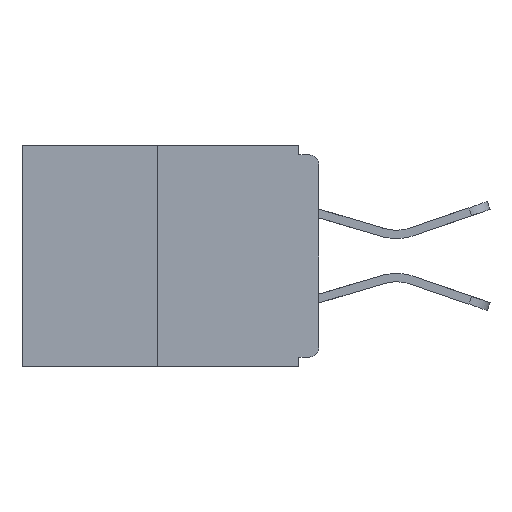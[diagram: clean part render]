
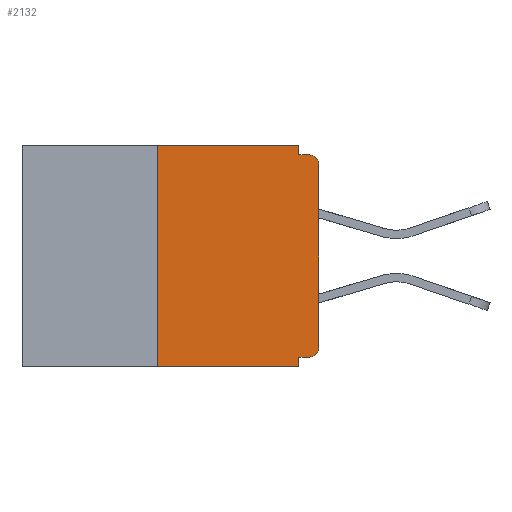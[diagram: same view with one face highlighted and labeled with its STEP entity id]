
A CAD part, left-side view. The second image highlights one B-rep face of the part: STEP entity #2132.
In plain terms, the highlighted planar face has unit normal (-1, 0, 0).
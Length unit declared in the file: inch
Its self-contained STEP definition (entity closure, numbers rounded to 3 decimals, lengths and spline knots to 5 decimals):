
#478 = ORIENTED_EDGE ( 'NONE', *, *, #6027, .F. ) ;
#513 = CARTESIAN_POINT ( 'NONE',  ( 0., 0., 0. ) ) ;
#827 = CARTESIAN_POINT ( 'NONE',  ( 0., 0.031, 0. ) ) ;
#1847 = CARTESIAN_POINT ( 'NONE',  ( 0., 0., -0.328 ) ) ;
#2132 = ADVANCED_FACE ( 'NONE', ( #8155 ), #9119, .F. ) ;
#2472 = ORIENTED_EDGE ( 'NONE', *, *, #11041, .F. ) ;
#3464 = CARTESIAN_POINT ( 'NONE',  ( 0., 0.46, 0. ) ) ;
#3646 = CARTESIAN_POINT ( 'NONE',  ( 0., 0.031, -0.015 ) ) ;
#4308 = VECTOR ( 'NONE', #7801, 39.37008 ) ;
#4330 = LINE ( 'NONE', #12150, #16354 ) ;
#4912 = EDGE_CURVE ( 'NONE', #11261, #14830, #19458, .T. ) ;
#5248 = ORIENTED_EDGE ( 'NONE', *, *, #5717, .F. ) ;
#5266 = LINE ( 'NONE', #8279, #11574 ) ;
#5592 = CARTESIAN_POINT ( 'NONE',  ( 0., 0.46, 0. ) ) ;
#5676 = DIRECTION ( 'NONE',  ( 0., -1., 0. ) ) ;
#5717 = EDGE_CURVE ( 'NONE', #6964, #14830, #18821, .T. ) ;
#6027 = EDGE_CURVE ( 'NONE', #24939, #6964, #5266, .T. ) ;
#6182 = DIRECTION ( 'NONE',  ( 0., 0., -1. ) ) ;
#6317 = DIRECTION ( 'NONE',  ( 0., 0., 1. ) ) ;
#6696 = VERTEX_POINT ( 'NONE', #16101 ) ;
#6715 = LINE ( 'NONE', #23277, #4308 ) ;
#6763 = DIRECTION ( 'NONE',  ( -1., 0., 0. ) ) ;
#6900 = VERTEX_POINT ( 'NONE', #21086 ) ;
#6964 = VERTEX_POINT ( 'NONE', #3646 ) ;
#7274 = DIRECTION ( 'NONE',  ( 0., 0., -1. ) ) ;
#7403 = VECTOR ( 'NONE', #16596, 39.37008 ) ;
#7737 = ORIENTED_EDGE ( 'NONE', *, *, #10737, .T. ) ;
#7801 = DIRECTION ( 'NONE',  ( 0., -1., 0. ) ) ;
#8001 = DIRECTION ( 'NONE',  ( 0., 0., -1. ) ) ;
#8126 = DIRECTION ( 'NONE',  ( 0., 0., -1. ) ) ;
#8155 = FACE_OUTER_BOUND ( 'NONE', #24048, .T. ) ;
#8279 = CARTESIAN_POINT ( 'NONE',  ( 0., 0.031, 0. ) ) ;
#8418 = VERTEX_POINT ( 'NONE', #11723 ) ;
#8738 = ORIENTED_EDGE ( 'NONE', *, *, #9827, .F. ) ;
#8752 = EDGE_CURVE ( 'NONE', #11117, #6696, #12344, .T. ) ;
#8955 = CARTESIAN_POINT ( 'NONE',  ( 0., 0., -0.015 ) ) ;
#9119 = PLANE ( 'NONE',  #12681 ) ;
#9827 = EDGE_CURVE ( 'NONE', #15967, #6900, #18626, .T. ) ;
#10737 = EDGE_CURVE ( 'NONE', #11117, #8418, #11955, .T. ) ;
#10884 = ORIENTED_EDGE ( 'NONE', *, *, #18009, .F. ) ;
#10940 = CARTESIAN_POINT ( 'NONE',  ( 0., 0.25, -0.343 ) ) ;
#11041 = EDGE_CURVE ( 'NONE', #6900, #24939, #11637, .T. ) ;
#11117 = VERTEX_POINT ( 'NONE', #15347 ) ;
#11261 = VERTEX_POINT ( 'NONE', #15743 ) ;
#11399 = VECTOR ( 'NONE', #14723, 39.37008 ) ;
#11574 = VECTOR ( 'NONE', #6182, 39.37008 ) ;
#11637 = LINE ( 'NONE', #5592, #21295 ) ;
#11723 = CARTESIAN_POINT ( 'NONE',  ( 0., 0., -0.313 ) ) ;
#11955 = CIRCLE ( 'NONE', #20068, 0.015 ) ;
#12150 = CARTESIAN_POINT ( 'NONE',  ( 0., 0.031, -0.343 ) ) ;
#12343 = LINE ( 'NONE', #513, #22923 ) ;
#12344 = LINE ( 'NONE', #1847, #23828 ) ;
#12681 = AXIS2_PLACEMENT_3D ( 'NONE', #3464, #12968, #7274 ) ;
#12968 = DIRECTION ( 'NONE',  ( 1., 0., 0. ) ) ;
#14162 = CARTESIAN_POINT ( 'NONE',  ( 0., 0.015, -0.313 ) ) ;
#14723 = DIRECTION ( 'NONE',  ( 0., 0., 1. ) ) ;
#14830 = VERTEX_POINT ( 'NONE', #24070 ) ;
#15347 = CARTESIAN_POINT ( 'NONE',  ( 0., 0.015, -0.328 ) ) ;
#15743 = CARTESIAN_POINT ( 'NONE',  ( 0., 0., -0.03 ) ) ;
#15967 = VERTEX_POINT ( 'NONE', #10940 ) ;
#16101 = CARTESIAN_POINT ( 'NONE',  ( 0., 0.031, -0.328 ) ) ;
#16354 = VECTOR ( 'NONE', #8126, 39.37008 ) ;
#16596 = DIRECTION ( 'NONE',  ( 0., -1., 0. ) ) ;
#17575 = AXIS2_PLACEMENT_3D ( 'NONE', #21307, #19428, #8001 ) ;
#17895 = EDGE_CURVE ( 'NONE', #15967, #18584, #6715, .T. ) ;
#18009 = EDGE_CURVE ( 'NONE', #6696, #18584, #4330, .T. ) ;
#18130 = ORIENTED_EDGE ( 'NONE', *, *, #19625, .T. ) ;
#18584 = VERTEX_POINT ( 'NONE', #20282 ) ;
#18610 = ORIENTED_EDGE ( 'NONE', *, *, #8752, .F. ) ;
#18626 = LINE ( 'NONE', #20621, #11399 ) ;
#18821 = LINE ( 'NONE', #8955, #7403 ) ;
#19428 = DIRECTION ( 'NONE',  ( -1., 0., 0. ) ) ;
#19458 = CIRCLE ( 'NONE', #17575, 0.015 ) ;
#19483 = ORIENTED_EDGE ( 'NONE', *, *, #4912, .T. ) ;
#19625 = EDGE_CURVE ( 'NONE', #8418, #11261, #12343, .T. ) ;
#20068 = AXIS2_PLACEMENT_3D ( 'NONE', #14162, #6763, #20220 ) ;
#20220 = DIRECTION ( 'NONE',  ( 0., 0., -1. ) ) ;
#20282 = CARTESIAN_POINT ( 'NONE',  ( 0., 0.031, -0.343 ) ) ;
#20621 = CARTESIAN_POINT ( 'NONE',  ( 0., 0.25, 0. ) ) ;
#21086 = CARTESIAN_POINT ( 'NONE',  ( 0., 0.25, 0. ) ) ;
#21295 = VECTOR ( 'NONE', #5676, 39.37008 ) ;
#21307 = CARTESIAN_POINT ( 'NONE',  ( 0., 0.015, -0.03 ) ) ;
#21974 = ORIENTED_EDGE ( 'NONE', *, *, #17895, .T. ) ;
#22923 = VECTOR ( 'NONE', #6317, 39.37008 ) ;
#23277 = CARTESIAN_POINT ( 'NONE',  ( 0., 0.46, -0.343 ) ) ;
#23828 = VECTOR ( 'NONE', #24761, 39.37008 ) ;
#24048 = EDGE_LOOP ( 'NONE', ( #2472, #8738, #21974, #10884, #18610, #7737, #18130, #19483, #5248, #478 ) ) ;
#24070 = CARTESIAN_POINT ( 'NONE',  ( 0., 0.015, -0.015 ) ) ;
#24761 = DIRECTION ( 'NONE',  ( 0., 1., 0. ) ) ;
#24939 = VERTEX_POINT ( 'NONE', #827 ) ;
